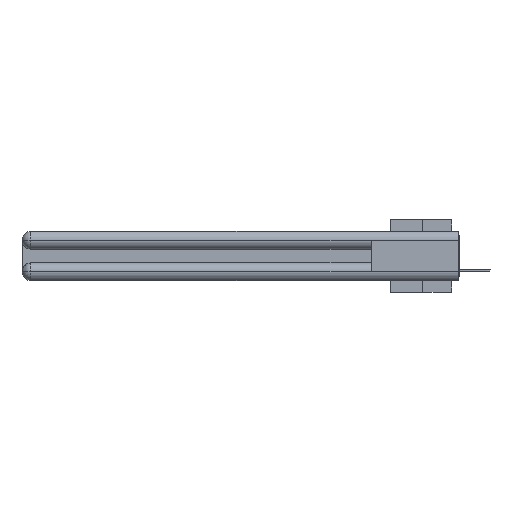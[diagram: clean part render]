
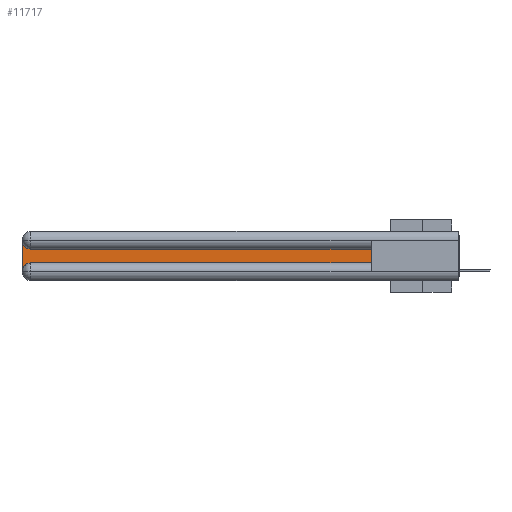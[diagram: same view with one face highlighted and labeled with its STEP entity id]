
A CAD part, left-side view. The second image highlights one B-rep face of the part: STEP entity #11717.
In plain terms, the highlighted planar face has unit normal (-1, 0, 0).
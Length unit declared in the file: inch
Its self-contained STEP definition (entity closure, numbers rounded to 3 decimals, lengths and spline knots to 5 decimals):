
#79 = DIRECTION ( 'NONE',  ( 0., 0., -1. ) ) ;
#428 = ORIENTED_EDGE ( 'NONE', *, *, #21119, .T. ) ;
#1797 = CARTESIAN_POINT ( 'NONE',  ( 0.075, 0.6, -0.1225 ) ) ;
#3553 = DIRECTION ( 'NONE',  ( 0., 0., -1. ) ) ;
#3814 = ORIENTED_EDGE ( 'NONE', *, *, #22539, .T. ) ;
#4198 = ORIENTED_EDGE ( 'NONE', *, *, #30348, .T. ) ;
#4312 = DIRECTION ( 'NONE',  ( 1., 0., 0. ) ) ;
#4511 = DIRECTION ( 'NONE',  ( 0., 0., -1. ) ) ;
#4942 = ORIENTED_EDGE ( 'NONE', *, *, #24018, .T. ) ;
#5336 = CIRCLE ( 'NONE', #22574, 0.06 ) ;
#6125 = CARTESIAN_POINT ( 'NONE',  ( 0.075, 3., -0.2175 ) ) ;
#6133 = VECTOR ( 'NONE', #21383, 39.37008 ) ;
#7174 = DIRECTION ( 'NONE',  ( 0., 0., 1. ) ) ;
#8793 = CARTESIAN_POINT ( 'NONE',  ( 0.075, 3., -0.0625 ) ) ;
#9257 = DIRECTION ( 'NONE',  ( 0., 1., 0. ) ) ;
#9259 = CIRCLE ( 'NONE', #13161, 0.06 ) ;
#10205 = FACE_OUTER_BOUND ( 'NONE', #19443, .T. ) ;
#11009 = LINE ( 'NONE', #24171, #31932 ) ;
#11017 = CARTESIAN_POINT ( 'NONE',  ( 0.075, 3., -0.2775 ) ) ;
#11717 = ADVANCED_FACE ( 'NONE', ( #10205 ), #32568, .F. ) ;
#11894 = VERTEX_POINT ( 'NONE', #27907 ) ;
#12865 = EDGE_CURVE ( 'NONE', #16644, #11894, #19607, .T. ) ;
#13161 = AXIS2_PLACEMENT_3D ( 'NONE', #19667, #4312, #4511 ) ;
#15012 = VECTOR ( 'NONE', #21683, 39.37008 ) ;
#15713 = VECTOR ( 'NONE', #7174, 39.37008 ) ;
#16644 = VERTEX_POINT ( 'NONE', #26258 ) ;
#17163 = EDGE_CURVE ( 'NONE', #24450, #32287, #23681, .T. ) ;
#19443 = EDGE_LOOP ( 'NONE', ( #428, #4198, #24184, #4942, #32068, #3814 ) ) ;
#19607 = LINE ( 'NONE', #23904, #6133 ) ;
#19667 = CARTESIAN_POINT ( 'NONE',  ( 0.075, 2.94, -0.2775 ) ) ;
#21023 = CARTESIAN_POINT ( 'NONE',  ( 0.075, 2.94, -0.0625 ) ) ;
#21119 = EDGE_CURVE ( 'NONE', #21851, #22599, #11009, .T. ) ;
#21383 = DIRECTION ( 'NONE',  ( 0., -1., 0. ) ) ;
#21683 = DIRECTION ( 'NONE',  ( 0., 0., -1. ) ) ;
#21851 = VERTEX_POINT ( 'NONE', #1797 ) ;
#22314 = CARTESIAN_POINT ( 'NONE',  ( 0.075, 3., -0.1225 ) ) ;
#22539 = EDGE_CURVE ( 'NONE', #11894, #21851, #27131, .T. ) ;
#22574 = AXIS2_PLACEMENT_3D ( 'NONE', #21023, #31263, #3553 ) ;
#22599 = VERTEX_POINT ( 'NONE', #25491 ) ;
#23681 = LINE ( 'NONE', #6125, #15012 ) ;
#23904 = CARTESIAN_POINT ( 'NONE',  ( 0.075, 0.6, -0.2175 ) ) ;
#24018 = EDGE_CURVE ( 'NONE', #32287, #16644, #9259, .T. ) ;
#24171 = CARTESIAN_POINT ( 'NONE',  ( 0.075, 0.6, -0.1225 ) ) ;
#24184 = ORIENTED_EDGE ( 'NONE', *, *, #17163, .T. ) ;
#24450 = VERTEX_POINT ( 'NONE', #8793 ) ;
#25348 = AXIS2_PLACEMENT_3D ( 'NONE', #22314, #30333, #79 ) ;
#25491 = CARTESIAN_POINT ( 'NONE',  ( 0.075, 2.94, -0.1225 ) ) ;
#26258 = CARTESIAN_POINT ( 'NONE',  ( 0.075, 2.94, -0.2175 ) ) ;
#27131 = LINE ( 'NONE', #32473, #15713 ) ;
#27907 = CARTESIAN_POINT ( 'NONE',  ( 0.075, 0.6, -0.2175 ) ) ;
#30333 = DIRECTION ( 'NONE',  ( 1., 0., 0. ) ) ;
#30348 = EDGE_CURVE ( 'NONE', #22599, #24450, #5336, .T. ) ;
#31263 = DIRECTION ( 'NONE',  ( 1., 0., 0. ) ) ;
#31932 = VECTOR ( 'NONE', #9257, 39.37008 ) ;
#32068 = ORIENTED_EDGE ( 'NONE', *, *, #12865, .T. ) ;
#32287 = VERTEX_POINT ( 'NONE', #11017 ) ;
#32473 = CARTESIAN_POINT ( 'NONE',  ( 0.075, 0.6, -0.2175 ) ) ;
#32568 = PLANE ( 'NONE',  #25348 ) ;
